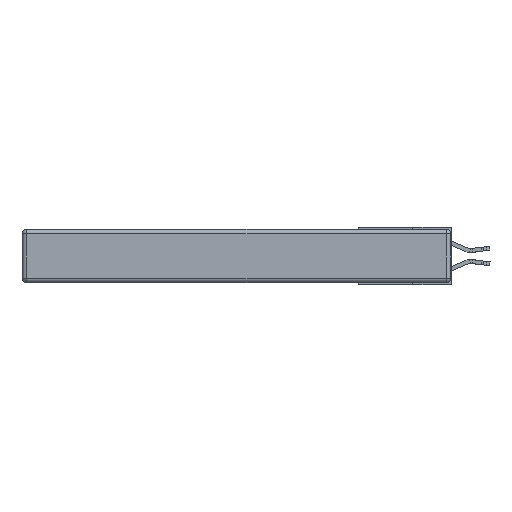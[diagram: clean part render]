
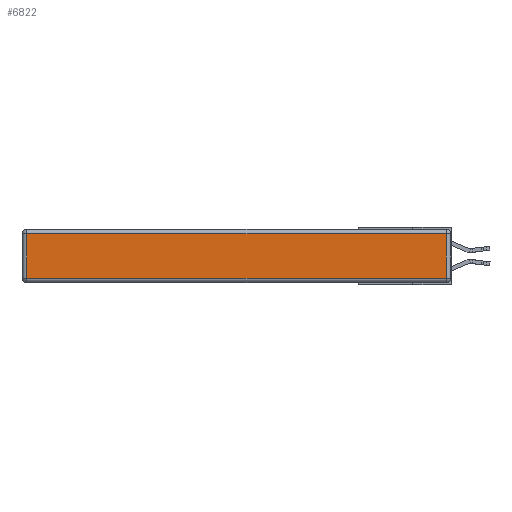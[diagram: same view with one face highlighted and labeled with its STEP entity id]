
A CAD part, left-side view. The second image highlights one B-rep face of the part: STEP entity #6822.
In plain terms, the highlighted planar face has unit normal (-1, 0, 0).
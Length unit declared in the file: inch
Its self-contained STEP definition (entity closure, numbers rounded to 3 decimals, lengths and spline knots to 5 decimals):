
#168 = VERTEX_POINT ( 'NONE', #28206 ) ;
#794 = DIRECTION ( 'NONE',  ( 0., 0., 1. ) ) ;
#3318 = CARTESIAN_POINT ( 'NONE',  ( 0., 2.72, -0.313 ) ) ;
#3589 = CARTESIAN_POINT ( 'NONE',  ( 0., 2.72, -0.03 ) ) ;
#5494 = EDGE_CURVE ( 'NONE', #30361, #34766, #18848, .T. ) ;
#6641 = VECTOR ( 'NONE', #25905, 39.37008 ) ;
#6710 = CARTESIAN_POINT ( 'NONE',  ( 0., 0., -0.343 ) ) ;
#6822 = ADVANCED_FACE ( 'NONE', ( #19164 ), #20131, .T. ) ;
#7600 = ORIENTED_EDGE ( 'NONE', *, *, #10072, .T. ) ;
#8775 = EDGE_CURVE ( 'NONE', #168, #30361, #26212, .T. ) ;
#10072 = EDGE_CURVE ( 'NONE', #34766, #11892, #12204, .T. ) ;
#11071 = CARTESIAN_POINT ( 'NONE',  ( 0., 0.03, -0.343 ) ) ;
#11892 = VERTEX_POINT ( 'NONE', #32593 ) ;
#12204 = LINE ( 'NONE', #22326, #30274 ) ;
#13728 = DIRECTION ( 'NONE',  ( 0., -1., 0. ) ) ;
#16019 = ORIENTED_EDGE ( 'NONE', *, *, #8775, .T. ) ;
#16433 = ORIENTED_EDGE ( 'NONE', *, *, #5494, .T. ) ;
#18347 = VECTOR ( 'NONE', #24871, 39.37008 ) ;
#18533 = ORIENTED_EDGE ( 'NONE', *, *, #23126, .T. ) ;
#18848 = LINE ( 'NONE', #20240, #6641 ) ;
#19164 = FACE_OUTER_BOUND ( 'NONE', #32369, .T. ) ;
#20131 = PLANE ( 'NONE',  #20673 ) ;
#20240 = CARTESIAN_POINT ( 'NONE',  ( 0., 2.72, -0.343 ) ) ;
#20673 = AXIS2_PLACEMENT_3D ( 'NONE', #6710, #22735, #794 ) ;
#22326 = CARTESIAN_POINT ( 'NONE',  ( 0., 0., -0.313 ) ) ;
#22735 = DIRECTION ( 'NONE',  ( -1., 0., 0. ) ) ;
#23126 = EDGE_CURVE ( 'NONE', #11892, #168, #25555, .T. ) ;
#24871 = DIRECTION ( 'NONE',  ( 0., 0., 1. ) ) ;
#25555 = LINE ( 'NONE', #11071, #18347 ) ;
#25905 = DIRECTION ( 'NONE',  ( 0., 0., -1. ) ) ;
#26212 = LINE ( 'NONE', #32078, #31345 ) ;
#28206 = CARTESIAN_POINT ( 'NONE',  ( 0., 0.03, -0.03 ) ) ;
#29176 = DIRECTION ( 'NONE',  ( 0., 1., 0. ) ) ;
#30274 = VECTOR ( 'NONE', #13728, 39.37008 ) ;
#30361 = VERTEX_POINT ( 'NONE', #3589 ) ;
#31345 = VECTOR ( 'NONE', #29176, 39.37008 ) ;
#32078 = CARTESIAN_POINT ( 'NONE',  ( 0., 2.75, -0.03 ) ) ;
#32369 = EDGE_LOOP ( 'NONE', ( #7600, #18533, #16019, #16433 ) ) ;
#32593 = CARTESIAN_POINT ( 'NONE',  ( 0., 0.03, -0.313 ) ) ;
#34766 = VERTEX_POINT ( 'NONE', #3318 ) ;
